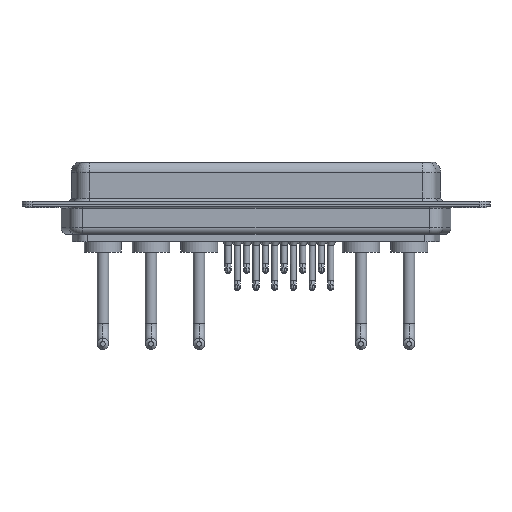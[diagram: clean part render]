
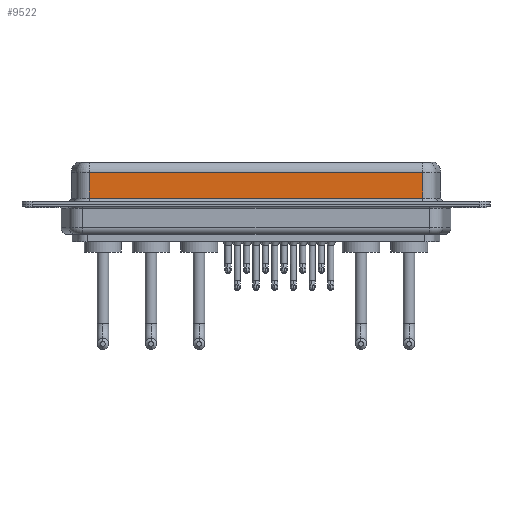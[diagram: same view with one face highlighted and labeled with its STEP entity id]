
A CAD part, front view. The second image highlights one B-rep face of the part: STEP entity #9522.
In plain terms, the highlighted planar face has unit normal (0, -1, 0).
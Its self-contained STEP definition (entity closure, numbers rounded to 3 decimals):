
#172 = CARTESIAN_POINT ( 'NONE',  ( 56.462, -3.95, 0.9 ) ) ;
#300 = CARTESIAN_POINT ( 'NONE',  ( 7.038, -3.95, 6.4 ) ) ;
#1401 = VECTOR ( 'NONE', #6264, 1000. ) ;
#1990 = FACE_OUTER_BOUND ( 'NONE', #14053, .T. ) ;
#4295 = ORIENTED_EDGE ( 'NONE', *, *, #15023, .T. ) ;
#4307 = LINE ( 'NONE', #4391, #6460 ) ;
#4391 = CARTESIAN_POINT ( 'NONE',  ( 56.462, -3.95, 0.9 ) ) ;
#5575 = CARTESIAN_POINT ( 'NONE',  ( 7.038, -3.95, 0.9 ) ) ;
#6235 = DIRECTION ( 'NONE',  ( 0., 0., -1. ) ) ;
#6264 = DIRECTION ( 'NONE',  ( -1., 0., 0. ) ) ;
#6359 = AXIS2_PLACEMENT_3D ( 'NONE', #12003, #10585, #17771 ) ;
#6460 = VECTOR ( 'NONE', #13101, 1000. ) ;
#7004 = CARTESIAN_POINT ( 'NONE',  ( 7.038, -3.95, 4.65 ) ) ;
#7244 = CARTESIAN_POINT ( 'NONE',  ( 56.462, -3.95, 4.65 ) ) ;
#7355 = EDGE_CURVE ( 'NONE', #13385, #17029, #7995, .T. ) ;
#7475 = DIRECTION ( 'NONE',  ( 0., 0., -1. ) ) ;
#7647 = LINE ( 'NONE', #300, #12766 ) ;
#7680 = PLANE ( 'NONE',  #6359 ) ;
#7932 = CARTESIAN_POINT ( 'NONE',  ( 56.462, -3.95, 4.65 ) ) ;
#7995 = LINE ( 'NONE', #14763, #8363 ) ;
#8363 = VECTOR ( 'NONE', #6235, 1000. ) ;
#8820 = VERTEX_POINT ( 'NONE', #5575 ) ;
#9522 = ADVANCED_FACE ( 'NONE', ( #1990 ), #7680, .F. ) ;
#9786 = ORIENTED_EDGE ( 'NONE', *, *, #7355, .F. ) ;
#10585 = DIRECTION ( 'NONE',  ( 0., 1., 0. ) ) ;
#10751 = LINE ( 'NONE', #7932, #1401 ) ;
#11772 = ORIENTED_EDGE ( 'NONE', *, *, #13910, .T. ) ;
#12003 = CARTESIAN_POINT ( 'NONE',  ( 56.462, -3.95, 6.4 ) ) ;
#12093 = ORIENTED_EDGE ( 'NONE', *, *, #13889, .T. ) ;
#12766 = VECTOR ( 'NONE', #7475, 1000. ) ;
#13101 = DIRECTION ( 'NONE',  ( 1., 0., 0. ) ) ;
#13385 = VERTEX_POINT ( 'NONE', #7244 ) ;
#13889 = EDGE_CURVE ( 'NONE', #8820, #17029, #4307, .T. ) ;
#13910 = EDGE_CURVE ( 'NONE', #13385, #17830, #10751, .T. ) ;
#14053 = EDGE_LOOP ( 'NONE', ( #9786, #11772, #4295, #12093 ) ) ;
#14763 = CARTESIAN_POINT ( 'NONE',  ( 56.462, -3.95, 6.4 ) ) ;
#15023 = EDGE_CURVE ( 'NONE', #17830, #8820, #7647, .T. ) ;
#17029 = VERTEX_POINT ( 'NONE', #172 ) ;
#17771 = DIRECTION ( 'NONE',  ( 0., 0., 1. ) ) ;
#17830 = VERTEX_POINT ( 'NONE', #7004 ) ;
